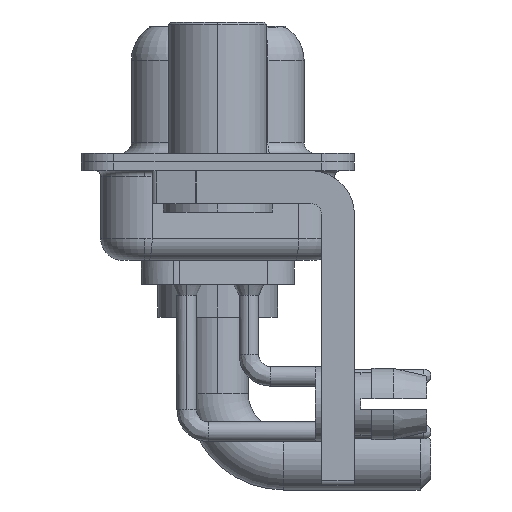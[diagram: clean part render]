
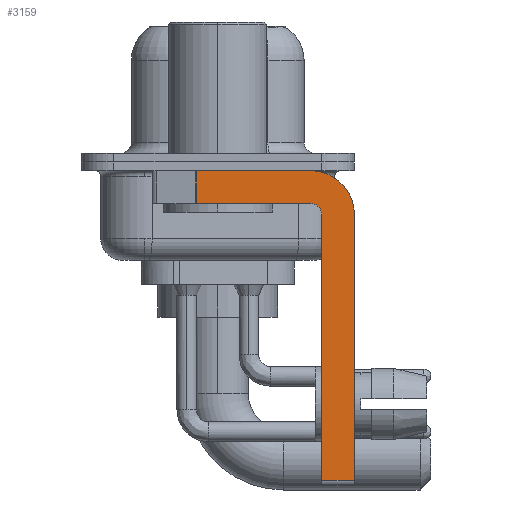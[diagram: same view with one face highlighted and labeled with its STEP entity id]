
A CAD part, left-side view. The second image highlights one B-rep face of the part: STEP entity #3159.
In plain terms, the highlighted planar face has unit normal (-1, 0, 0).
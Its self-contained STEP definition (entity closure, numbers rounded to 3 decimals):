
#1244 = DIRECTION ( 'NONE',  ( 0., 0., 1. ) ) ;
#1391 = EDGE_CURVE ( 'NONE', #18287, #1541, #10849, .T. ) ;
#1541 = VERTEX_POINT ( 'NONE', #1719 ) ;
#1660 = CARTESIAN_POINT ( 'NONE',  ( -2.9, 3., -0.4 ) ) ;
#1719 = CARTESIAN_POINT ( 'NONE',  ( -2.9, -4.25, -1.9 ) ) ;
#2102 = EDGE_CURVE ( 'NONE', #16085, #18287, #4677, .T. ) ;
#2509 = EDGE_CURVE ( 'NONE', #16085, #4267, #8281, .T. ) ;
#2998 = VERTEX_POINT ( 'NONE', #16776 ) ;
#3085 = DIRECTION ( 'NONE',  ( -1., 0., 0. ) ) ;
#3159 = ADVANCED_FACE ( 'NONE', ( #17578 ), #8896, .F. ) ;
#3163 = VERTEX_POINT ( 'NONE', #15527 ) ;
#4137 = ORIENTED_EDGE ( 'NONE', *, *, #15399, .F. ) ;
#4258 = CARTESIAN_POINT ( 'NONE',  ( -2.9, 0.978, -0.4 ) ) ;
#4267 = VERTEX_POINT ( 'NONE', #9859 ) ;
#4677 = LINE ( 'NONE', #21810, #18321 ) ;
#4928 = EDGE_CURVE ( 'NONE', #5639, #7445, #7049, .T. ) ;
#5617 = DIRECTION ( 'NONE',  ( 0., 0., -1. ) ) ;
#5639 = VERTEX_POINT ( 'NONE', #4258 ) ;
#5797 = DIRECTION ( 'NONE',  ( 0., 1., 0. ) ) ;
#6800 = LINE ( 'NONE', #1660, #21637 ) ;
#6860 = DIRECTION ( 'NONE',  ( 0., 0., 1. ) ) ;
#7049 = LINE ( 'NONE', #13911, #21077 ) ;
#7276 = DIRECTION ( 'NONE',  ( 1., 0., 0. ) ) ;
#7445 = VERTEX_POINT ( 'NONE', #18501 ) ;
#8281 = LINE ( 'NONE', #18356, #10429 ) ;
#8896 = PLANE ( 'NONE',  #12431 ) ;
#9859 = CARTESIAN_POINT ( 'NONE',  ( -2.9, -6.25, -14.55 ) ) ;
#9919 = VECTOR ( 'NONE', #5797, 1000. ) ;
#10115 = ORIENTED_EDGE ( 'NONE', *, *, #1391, .F. ) ;
#10429 = VECTOR ( 'NONE', #15040, 1000. ) ;
#10491 = ORIENTED_EDGE ( 'NONE', *, *, #11588, .F. ) ;
#10792 = ORIENTED_EDGE ( 'NONE', *, *, #15879, .F. ) ;
#10849 = CIRCLE ( 'NONE', #18890, 0.5 ) ;
#11588 = EDGE_CURVE ( 'NONE', #3163, #4267, #14650, .T. ) ;
#11773 = CARTESIAN_POINT ( 'NONE',  ( -2.9, -4.25, -2.4 ) ) ;
#11881 = DIRECTION ( 'NONE',  ( 1., 0., 0. ) ) ;
#12181 = CARTESIAN_POINT ( 'NONE',  ( -2.9, -4.75, -2.4 ) ) ;
#12431 = AXIS2_PLACEMENT_3D ( 'NONE', #15861, #7276, #20683 ) ;
#12946 = ORIENTED_EDGE ( 'NONE', *, *, #14802, .F. ) ;
#13230 = CIRCLE ( 'NONE', #18698, 2. ) ;
#13776 = DIRECTION ( 'NONE',  ( 0., -1., 0. ) ) ;
#13890 = VECTOR ( 'NONE', #5617, 1000. ) ;
#13911 = CARTESIAN_POINT ( 'NONE',  ( -2.9, 0.978, -1.9 ) ) ;
#14650 = LINE ( 'NONE', #19815, #13890 ) ;
#14802 = EDGE_CURVE ( 'NONE', #1541, #7445, #16411, .T. ) ;
#15040 = DIRECTION ( 'NONE',  ( 0., -1., 0. ) ) ;
#15318 = CARTESIAN_POINT ( 'NONE',  ( -2.9, -4.25, -2.4 ) ) ;
#15399 = EDGE_CURVE ( 'NONE', #2998, #3163, #13230, .T. ) ;
#15527 = CARTESIAN_POINT ( 'NONE',  ( -2.9, -6.25, -2.4 ) ) ;
#15861 = CARTESIAN_POINT ( 'NONE',  ( -2.9, -4.25, -2.4 ) ) ;
#15879 = EDGE_CURVE ( 'NONE', #5639, #2998, #6800, .T. ) ;
#16085 = VERTEX_POINT ( 'NONE', #21757 ) ;
#16411 = LINE ( 'NONE', #21463, #9919 ) ;
#16776 = CARTESIAN_POINT ( 'NONE',  ( -2.9, -4.25, -0.4 ) ) ;
#17009 = ORIENTED_EDGE ( 'NONE', *, *, #2102, .F. ) ;
#17578 = FACE_OUTER_BOUND ( 'NONE', #21387, .T. ) ;
#18287 = VERTEX_POINT ( 'NONE', #12181 ) ;
#18321 = VECTOR ( 'NONE', #1244, 1000. ) ;
#18356 = CARTESIAN_POINT ( 'NONE',  ( -2.9, -4.25, -14.55 ) ) ;
#18501 = CARTESIAN_POINT ( 'NONE',  ( -2.9, 0.978, -1.9 ) ) ;
#18698 = AXIS2_PLACEMENT_3D ( 'NONE', #11773, #11881, #18726 ) ;
#18726 = DIRECTION ( 'NONE',  ( 0., 0., -1. ) ) ;
#18890 = AXIS2_PLACEMENT_3D ( 'NONE', #15318, #3085, #6860 ) ;
#19815 = CARTESIAN_POINT ( 'NONE',  ( -2.9, -6.25, -2.4 ) ) ;
#20145 = ORIENTED_EDGE ( 'NONE', *, *, #2509, .T. ) ;
#20683 = DIRECTION ( 'NONE',  ( 0., 0., -1. ) ) ;
#20879 = ORIENTED_EDGE ( 'NONE', *, *, #4928, .T. ) ;
#21077 = VECTOR ( 'NONE', #21214, 1000. ) ;
#21214 = DIRECTION ( 'NONE',  ( 0., 0., -1. ) ) ;
#21387 = EDGE_LOOP ( 'NONE', ( #10792, #20879, #12946, #10115, #17009, #20145, #10491, #4137 ) ) ;
#21463 = CARTESIAN_POINT ( 'NONE',  ( -2.9, -4.25, -1.9 ) ) ;
#21637 = VECTOR ( 'NONE', #13776, 1000. ) ;
#21757 = CARTESIAN_POINT ( 'NONE',  ( -2.9, -4.75, -14.55 ) ) ;
#21810 = CARTESIAN_POINT ( 'NONE',  ( -2.9, -4.75, -14.8 ) ) ;
